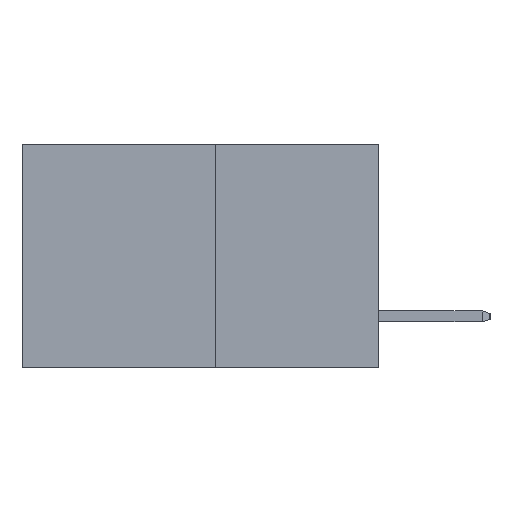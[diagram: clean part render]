
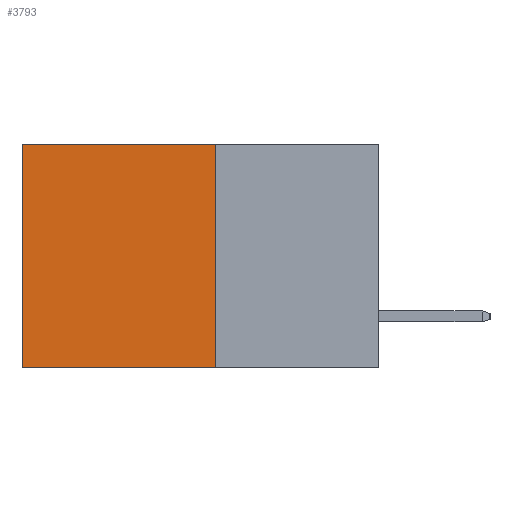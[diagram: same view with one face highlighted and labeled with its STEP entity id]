
A CAD part, left-side view. The second image highlights one B-rep face of the part: STEP entity #3793.
In plain terms, the highlighted planar face has unit normal (-1, 0, 0).
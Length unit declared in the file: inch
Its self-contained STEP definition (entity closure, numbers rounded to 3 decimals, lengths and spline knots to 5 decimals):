
#116 = AXIS2_PLACEMENT_3D ( 'NONE', #6831, #6903, #7568 ) ;
#186 = FACE_OUTER_BOUND ( 'NONE', #6124, .T. ) ;
#397 = VECTOR ( 'NONE', #7597, 39.37008 ) ;
#414 = DIRECTION ( 'NONE',  ( 0., 0., -1. ) ) ;
#650 = EDGE_CURVE ( 'NONE', #6092, #702, #3689, .T. ) ;
#702 = VERTEX_POINT ( 'NONE', #1098 ) ;
#763 = VERTEX_POINT ( 'NONE', #7747 ) ;
#958 = CARTESIAN_POINT ( 'NONE',  ( 0.277, 0.27, -0.37 ) ) ;
#1098 = CARTESIAN_POINT ( 'NONE',  ( 0.277, 0.59, -0.37 ) ) ;
#1445 = EDGE_CURVE ( 'NONE', #763, #7169, #3676, .T. ) ;
#2189 = LINE ( 'NONE', #3791, #3969 ) ;
#3676 = LINE ( 'NONE', #958, #8184 ) ;
#3689 = LINE ( 'NONE', #4938, #5003 ) ;
#3771 = ORIENTED_EDGE ( 'NONE', *, *, #650, .T. ) ;
#3786 = DIRECTION ( 'NONE',  ( 0., 1., 0. ) ) ;
#3791 = CARTESIAN_POINT ( 'NONE',  ( 0.277, 0.27, -0.37 ) ) ;
#3793 = ADVANCED_FACE ( 'NONE', ( #186 ), #5683, .F. ) ;
#3969 = VECTOR ( 'NONE', #3786, 39.37008 ) ;
#4092 = ORIENTED_EDGE ( 'NONE', *, *, #5518, .F. ) ;
#4612 = CARTESIAN_POINT ( 'NONE',  ( 0.277, 0.59, 0. ) ) ;
#4717 = CARTESIAN_POINT ( 'NONE',  ( 0.277, 0.27, -0.37 ) ) ;
#4938 = CARTESIAN_POINT ( 'NONE',  ( 0.277, 0.59, -0.37 ) ) ;
#4986 = ORIENTED_EDGE ( 'NONE', *, *, #1445, .F. ) ;
#4987 = EDGE_CURVE ( 'NONE', #763, #6092, #5672, .T. ) ;
#5003 = VECTOR ( 'NONE', #7288, 39.37008 ) ;
#5518 = EDGE_CURVE ( 'NONE', #7169, #702, #2189, .T. ) ;
#5672 = LINE ( 'NONE', #7632, #397 ) ;
#5683 = PLANE ( 'NONE',  #116 ) ;
#6092 = VERTEX_POINT ( 'NONE', #4612 ) ;
#6124 = EDGE_LOOP ( 'NONE', ( #3771, #4092, #4986, #6598 ) ) ;
#6598 = ORIENTED_EDGE ( 'NONE', *, *, #4987, .T. ) ;
#6831 = CARTESIAN_POINT ( 'NONE',  ( 0.277, 0.27, -0.37 ) ) ;
#6903 = DIRECTION ( 'NONE',  ( 1., 0., 0. ) ) ;
#7169 = VERTEX_POINT ( 'NONE', #4717 ) ;
#7288 = DIRECTION ( 'NONE',  ( 0., 0., -1. ) ) ;
#7568 = DIRECTION ( 'NONE',  ( 0., 0., -1. ) ) ;
#7597 = DIRECTION ( 'NONE',  ( 0., 1., 0. ) ) ;
#7632 = CARTESIAN_POINT ( 'NONE',  ( 0.277, 0.27, 0. ) ) ;
#7747 = CARTESIAN_POINT ( 'NONE',  ( 0.277, 0.27, 0. ) ) ;
#8184 = VECTOR ( 'NONE', #414, 39.37008 ) ;
